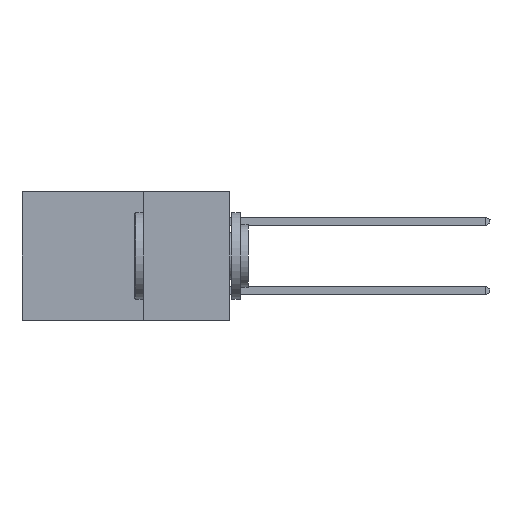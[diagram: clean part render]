
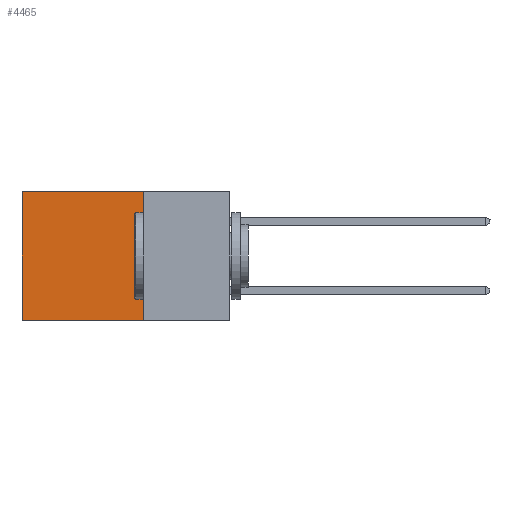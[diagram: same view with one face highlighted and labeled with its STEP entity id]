
A CAD part, left-side view. The second image highlights one B-rep face of the part: STEP entity #4465.
In plain terms, the highlighted planar face has unit normal (-1, 0, 0).
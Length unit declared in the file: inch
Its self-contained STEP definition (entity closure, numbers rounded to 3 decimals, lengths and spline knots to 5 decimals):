
#1001 = VECTOR ( 'NONE', #9455, 39.37008 ) ;
#1006 = VECTOR ( 'NONE', #21092, 39.37008 ) ;
#1139 = ORIENTED_EDGE ( 'NONE', *, *, #18102, .T. ) ;
#1505 = CARTESIAN_POINT ( 'NONE',  ( 0.298, 0.25, -0.37 ) ) ;
#2314 = CARTESIAN_POINT ( 'NONE',  ( 0.298, 0.6, 0. ) ) ;
#2370 = CARTESIAN_POINT ( 'NONE',  ( 0.298, 0.6, 0. ) ) ;
#2794 = CARTESIAN_POINT ( 'NONE',  ( 0.298, 0.25, 0. ) ) ;
#3145 = LINE ( 'NONE', #21862, #13452 ) ;
#4465 = ADVANCED_FACE ( 'NONE', ( #24810 ), #6179, .F. ) ;
#5027 = VERTEX_POINT ( 'NONE', #1505 ) ;
#5196 = EDGE_CURVE ( 'NONE', #12286, #16533, #3145, .T. ) ;
#5759 = DIRECTION ( 'NONE',  ( 0., 0., -1. ) ) ;
#5816 = DIRECTION ( 'NONE',  ( 1., 0., 0. ) ) ;
#6116 = CARTESIAN_POINT ( 'NONE',  ( 0.298, 0.25, 0. ) ) ;
#6179 = PLANE ( 'NONE',  #13997 ) ;
#7413 = CARTESIAN_POINT ( 'NONE',  ( 0.298, 0.25, 0. ) ) ;
#8968 = CARTESIAN_POINT ( 'NONE',  ( 0.298, 0.6, -0.37 ) ) ;
#9264 = DIRECTION ( 'NONE',  ( 0., 1., 0. ) ) ;
#9455 = DIRECTION ( 'NONE',  ( 0., 0., -1. ) ) ;
#9817 = EDGE_CURVE ( 'NONE', #12286, #5027, #12673, .T. ) ;
#10679 = ORIENTED_EDGE ( 'NONE', *, *, #9817, .F. ) ;
#12286 = VERTEX_POINT ( 'NONE', #2794 ) ;
#12673 = LINE ( 'NONE', #7413, #1001 ) ;
#13266 = ORIENTED_EDGE ( 'NONE', *, *, #5196, .T. ) ;
#13404 = EDGE_LOOP ( 'NONE', ( #1139, #17101, #10679, #13266 ) ) ;
#13452 = VECTOR ( 'NONE', #9264, 39.37008 ) ;
#13997 = AXIS2_PLACEMENT_3D ( 'NONE', #6116, #5816, #5759 ) ;
#15328 = EDGE_CURVE ( 'NONE', #5027, #17949, #15420, .T. ) ;
#15420 = LINE ( 'NONE', #21538, #25736 ) ;
#16533 = VERTEX_POINT ( 'NONE', #2314 ) ;
#17101 = ORIENTED_EDGE ( 'NONE', *, *, #15328, .F. ) ;
#17504 = LINE ( 'NONE', #2370, #1006 ) ;
#17949 = VERTEX_POINT ( 'NONE', #8968 ) ;
#18102 = EDGE_CURVE ( 'NONE', #16533, #17949, #17504, .T. ) ;
#21092 = DIRECTION ( 'NONE',  ( 0., 0., -1. ) ) ;
#21538 = CARTESIAN_POINT ( 'NONE',  ( 0.298, 0.25, -0.37 ) ) ;
#21862 = CARTESIAN_POINT ( 'NONE',  ( 0.298, 0.25, 0. ) ) ;
#23596 = DIRECTION ( 'NONE',  ( 0., 1., 0. ) ) ;
#24810 = FACE_OUTER_BOUND ( 'NONE', #13404, .T. ) ;
#25736 = VECTOR ( 'NONE', #23596, 39.37008 ) ;
